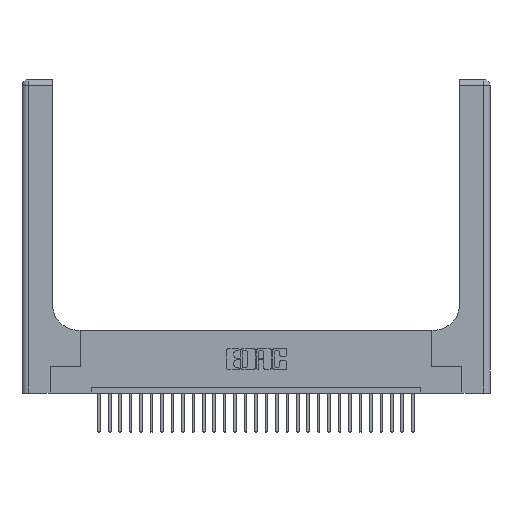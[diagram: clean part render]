
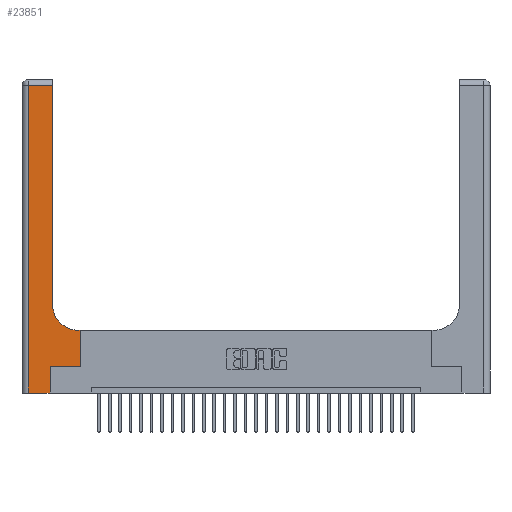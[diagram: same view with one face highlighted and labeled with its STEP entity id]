
A CAD part, top view. The second image highlights one B-rep face of the part: STEP entity #23851.
In plain terms, the highlighted planar face has unit normal (0, 0, 1).
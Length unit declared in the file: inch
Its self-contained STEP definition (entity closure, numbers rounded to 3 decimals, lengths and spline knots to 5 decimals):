
#81 = DIRECTION ( 'NONE',  ( 1., 0., 0. ) ) ;
#181 = VECTOR ( 'NONE', #20969, 39.37008 ) ;
#443 = VECTOR ( 'NONE', #22829, 39.37008 ) ;
#1231 = VECTOR ( 'NONE', #15629, 39.37008 ) ;
#1631 = LINE ( 'NONE', #13415, #12438 ) ;
#1902 = CARTESIAN_POINT ( 'NONE',  ( 0.06, 0., 0.37 ) ) ;
#1957 = LINE ( 'NONE', #29536, #1231 ) ;
#2092 = ORIENTED_EDGE ( 'NONE', *, *, #6257, .T. ) ;
#2523 = DIRECTION ( 'NONE',  ( 0., 0., -1. ) ) ;
#2541 = ORIENTED_EDGE ( 'NONE', *, *, #21717, .T. ) ;
#3030 = CARTESIAN_POINT ( 'NONE',  ( 0.5585, 0.6, 0.37 ) ) ;
#3203 = VERTEX_POINT ( 'NONE', #11956 ) ;
#3836 = CARTESIAN_POINT ( 'NONE',  ( 0.2915, 3., 0.37 ) ) ;
#3882 = CARTESIAN_POINT ( 'NONE',  ( 0., 3., 0.37 ) ) ;
#4993 = EDGE_CURVE ( 'NONE', #27872, #3203, #1957, .T. ) ;
#5021 = CARTESIAN_POINT ( 'NONE',  ( 0., 2.94, 0.37 ) ) ;
#5321 = VERTEX_POINT ( 'NONE', #3030 ) ;
#5848 = EDGE_LOOP ( 'NONE', ( #23102, #19636, #21683, #20784, #13912, #25522, #2541, #10866, #2092 ) ) ;
#6060 = CARTESIAN_POINT ( 'NONE',  ( 0.2915, 0.6, 0.37 ) ) ;
#6257 = EDGE_CURVE ( 'NONE', #16827, #9402, #21058, .T. ) ;
#6616 = CARTESIAN_POINT ( 'NONE',  ( 0., 0., 0.37 ) ) ;
#6799 = EDGE_CURVE ( 'NONE', #9402, #16319, #27903, .T. ) ;
#6852 = CARTESIAN_POINT ( 'NONE',  ( 0.269, 0.25, 0.37 ) ) ;
#7055 = CARTESIAN_POINT ( 'NONE',  ( 0.5415, 0.85, 0.37 ) ) ;
#7067 = LINE ( 'NONE', #5021, #181 ) ;
#8399 = DIRECTION ( 'NONE',  ( -1., 0., 0. ) ) ;
#8622 = AXIS2_PLACEMENT_3D ( 'NONE', #3882, #8641, #24462 ) ;
#8641 = DIRECTION ( 'NONE',  ( 0., 0., -1. ) ) ;
#8774 = CARTESIAN_POINT ( 'NONE',  ( 0.5585, 0.25, 0.37 ) ) ;
#8798 = LINE ( 'NONE', #6616, #443 ) ;
#9402 = VERTEX_POINT ( 'NONE', #21642 ) ;
#10756 = PLANE ( 'NONE',  #8622 ) ;
#10866 = ORIENTED_EDGE ( 'NONE', *, *, #16158, .T. ) ;
#11151 = DIRECTION ( 'NONE',  ( 0., -1., 0. ) ) ;
#11588 = CARTESIAN_POINT ( 'NONE',  ( 0.5415, 0.6, 0.37 ) ) ;
#11956 = CARTESIAN_POINT ( 'NONE',  ( 0.5585, 0.25, 0.37 ) ) ;
#12438 = VECTOR ( 'NONE', #27222, 39.37008 ) ;
#12923 = CARTESIAN_POINT ( 'NONE',  ( 0.2915, 2.94, 0.37 ) ) ;
#13415 = CARTESIAN_POINT ( 'NONE',  ( 0.269, 0., 0.37 ) ) ;
#13640 = LINE ( 'NONE', #17987, #24534 ) ;
#13912 = ORIENTED_EDGE ( 'NONE', *, *, #25780, .T. ) ;
#15629 = DIRECTION ( 'NONE',  ( 1., 0., 0. ) ) ;
#16158 = EDGE_CURVE ( 'NONE', #5321, #16827, #18372, .T. ) ;
#16319 = VERTEX_POINT ( 'NONE', #12923 ) ;
#16662 = VERTEX_POINT ( 'NONE', #16844 ) ;
#16827 = VERTEX_POINT ( 'NONE', #11588 ) ;
#16844 = CARTESIAN_POINT ( 'NONE',  ( 0.269, 0., 0.37 ) ) ;
#17705 = VERTEX_POINT ( 'NONE', #24886 ) ;
#17987 = CARTESIAN_POINT ( 'NONE',  ( 0.06, 3., 0.37 ) ) ;
#18372 = LINE ( 'NONE', #6060, #20552 ) ;
#19636 = ORIENTED_EDGE ( 'NONE', *, *, #24817, .T. ) ;
#20327 = VECTOR ( 'NONE', #29069, 39.37008 ) ;
#20552 = VECTOR ( 'NONE', #8399, 39.37008 ) ;
#20784 = ORIENTED_EDGE ( 'NONE', *, *, #26585, .T. ) ;
#20969 = DIRECTION ( 'NONE',  ( -1., 0., 0. ) ) ;
#21058 = CIRCLE ( 'NONE', #25140, 0.25 ) ;
#21642 = CARTESIAN_POINT ( 'NONE',  ( 0.2915, 0.85, 0.37 ) ) ;
#21683 = ORIENTED_EDGE ( 'NONE', *, *, #23916, .T. ) ;
#21717 = EDGE_CURVE ( 'NONE', #3203, #5321, #24326, .T. ) ;
#22190 = VERTEX_POINT ( 'NONE', #1902 ) ;
#22829 = DIRECTION ( 'NONE',  ( 1., 0., 0. ) ) ;
#23102 = ORIENTED_EDGE ( 'NONE', *, *, #6799, .T. ) ;
#23851 = ADVANCED_FACE ( 'NONE', ( #27074 ), #10756, .F. ) ;
#23916 = EDGE_CURVE ( 'NONE', #17705, #22190, #13640, .T. ) ;
#24326 = LINE ( 'NONE', #8774, #29035 ) ;
#24462 = DIRECTION ( 'NONE',  ( -1., 0., 0. ) ) ;
#24534 = VECTOR ( 'NONE', #11151, 39.37008 ) ;
#24817 = EDGE_CURVE ( 'NONE', #16319, #17705, #7067, .T. ) ;
#24886 = CARTESIAN_POINT ( 'NONE',  ( 0.06, 2.94, 0.37 ) ) ;
#25140 = AXIS2_PLACEMENT_3D ( 'NONE', #7055, #2523, #81 ) ;
#25522 = ORIENTED_EDGE ( 'NONE', *, *, #4993, .T. ) ;
#25780 = EDGE_CURVE ( 'NONE', #16662, #27872, #1631, .T. ) ;
#26585 = EDGE_CURVE ( 'NONE', #22190, #16662, #8798, .T. ) ;
#27074 = FACE_OUTER_BOUND ( 'NONE', #5848, .T. ) ;
#27222 = DIRECTION ( 'NONE',  ( 0., 1., 0. ) ) ;
#27872 = VERTEX_POINT ( 'NONE', #6852 ) ;
#27903 = LINE ( 'NONE', #3836, #20327 ) ;
#29035 = VECTOR ( 'NONE', #29764, 39.37008 ) ;
#29069 = DIRECTION ( 'NONE',  ( 0., 1., 0. ) ) ;
#29536 = CARTESIAN_POINT ( 'NONE',  ( 0.269, 0.25, 0.37 ) ) ;
#29764 = DIRECTION ( 'NONE',  ( 0., 1., 0. ) ) ;
